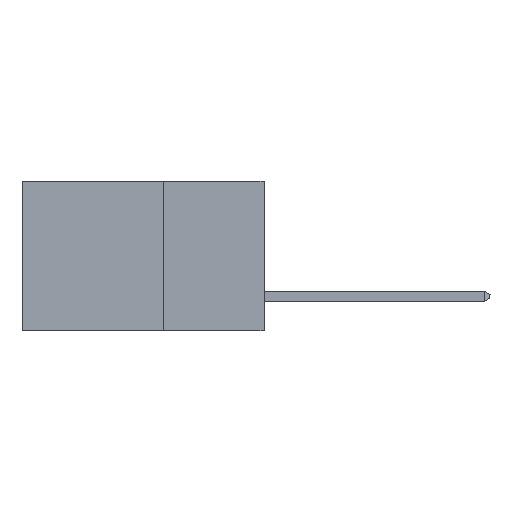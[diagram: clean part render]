
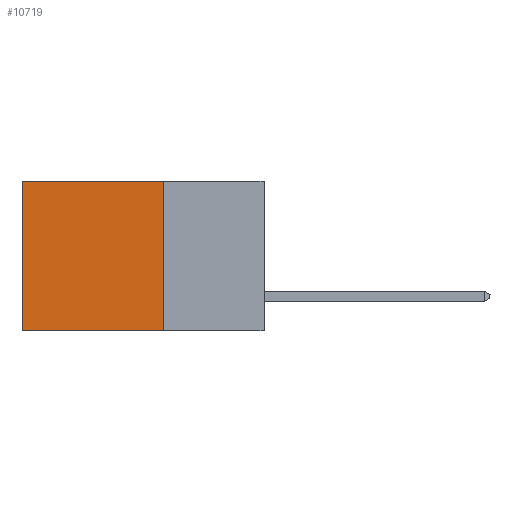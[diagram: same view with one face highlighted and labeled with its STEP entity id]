
A CAD part, left-side view. The second image highlights one B-rep face of the part: STEP entity #10719.
In plain terms, the highlighted planar face has unit normal (-1, 0, 0).
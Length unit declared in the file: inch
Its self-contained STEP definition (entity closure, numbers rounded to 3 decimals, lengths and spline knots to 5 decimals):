
#210 = CARTESIAN_POINT ( 'NONE',  ( 0.298, 0.25, 0. ) ) ;
#321 = VERTEX_POINT ( 'NONE', #1656 ) ;
#1656 = CARTESIAN_POINT ( 'NONE',  ( 0.298, 0.6, -0.37 ) ) ;
#2063 = VECTOR ( 'NONE', #8964, 39.37008 ) ;
#2316 = VECTOR ( 'NONE', #4728, 39.37008 ) ;
#2477 = CARTESIAN_POINT ( 'NONE',  ( 0.298, 0.25, -0.37 ) ) ;
#2515 = VECTOR ( 'NONE', #23938, 39.37008 ) ;
#2715 = LINE ( 'NONE', #16244, #2316 ) ;
#2887 = VERTEX_POINT ( 'NONE', #23078 ) ;
#3056 = AXIS2_PLACEMENT_3D ( 'NONE', #210, #12412, #17171 ) ;
#3757 = ORIENTED_EDGE ( 'NONE', *, *, #11085, .T. ) ;
#4728 = DIRECTION ( 'NONE',  ( 0., 1., 0. ) ) ;
#4884 = VERTEX_POINT ( 'NONE', #15331 ) ;
#5912 = EDGE_CURVE ( 'NONE', #4884, #21026, #22329, .T. ) ;
#6167 = VECTOR ( 'NONE', #10073, 39.37008 ) ;
#7737 = CARTESIAN_POINT ( 'NONE',  ( 0.298, 0.6, 0. ) ) ;
#8964 = DIRECTION ( 'NONE',  ( 0., 0., -1. ) ) ;
#9970 = CARTESIAN_POINT ( 'NONE',  ( 0.298, 0.25, -0.37 ) ) ;
#10073 = DIRECTION ( 'NONE',  ( 0., 1., 0. ) ) ;
#10192 = LINE ( 'NONE', #7737, #2515 ) ;
#10719 = ADVANCED_FACE ( 'NONE', ( #24948 ), #27916, .F. ) ;
#11085 = EDGE_CURVE ( 'NONE', #4884, #2887, #2715, .T. ) ;
#12412 = DIRECTION ( 'NONE',  ( 1., 0., 0. ) ) ;
#12470 = ORIENTED_EDGE ( 'NONE', *, *, #5912, .F. ) ;
#13135 = EDGE_CURVE ( 'NONE', #2887, #321, #10192, .T. ) ;
#15298 = ORIENTED_EDGE ( 'NONE', *, *, #13135, .T. ) ;
#15331 = CARTESIAN_POINT ( 'NONE',  ( 0.298, 0.25, 0. ) ) ;
#16244 = CARTESIAN_POINT ( 'NONE',  ( 0.298, 0.25, 0. ) ) ;
#16971 = EDGE_CURVE ( 'NONE', #21026, #321, #25259, .T. ) ;
#17171 = DIRECTION ( 'NONE',  ( 0., 0., -1. ) ) ;
#19195 = ORIENTED_EDGE ( 'NONE', *, *, #16971, .F. ) ;
#21026 = VERTEX_POINT ( 'NONE', #2477 ) ;
#21808 = EDGE_LOOP ( 'NONE', ( #15298, #19195, #12470, #3757 ) ) ;
#22329 = LINE ( 'NONE', #29430, #2063 ) ;
#23078 = CARTESIAN_POINT ( 'NONE',  ( 0.298, 0.6, 0. ) ) ;
#23938 = DIRECTION ( 'NONE',  ( 0., 0., -1. ) ) ;
#24948 = FACE_OUTER_BOUND ( 'NONE', #21808, .T. ) ;
#25259 = LINE ( 'NONE', #9970, #6167 ) ;
#27916 = PLANE ( 'NONE',  #3056 ) ;
#29430 = CARTESIAN_POINT ( 'NONE',  ( 0.298, 0.25, 0. ) ) ;
